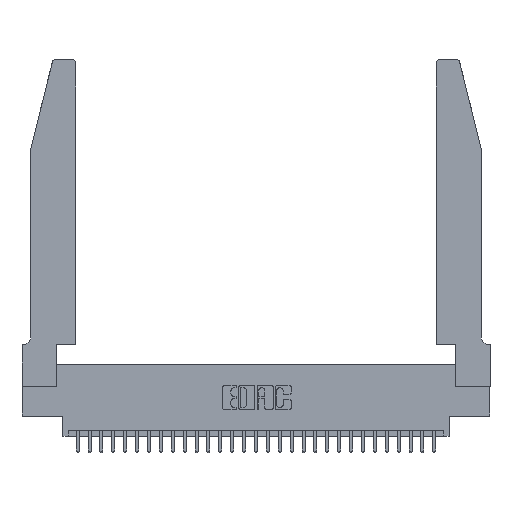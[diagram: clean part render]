
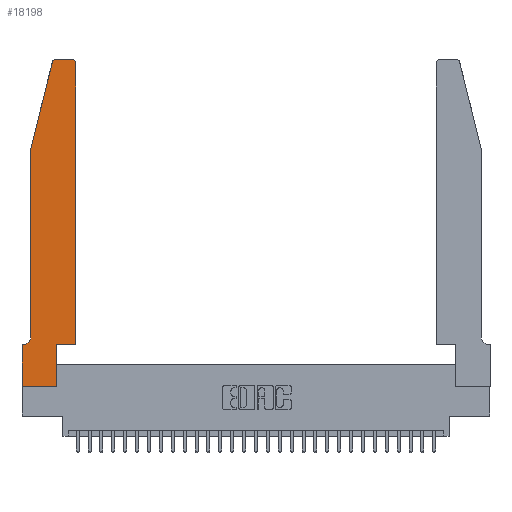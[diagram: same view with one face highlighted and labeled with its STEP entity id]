
A CAD part, top view. The second image highlights one B-rep face of the part: STEP entity #18198.
In plain terms, the highlighted planar face has unit normal (0, 0, 1).
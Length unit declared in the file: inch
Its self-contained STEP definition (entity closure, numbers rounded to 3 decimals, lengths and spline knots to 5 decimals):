
#87 = ORIENTED_EDGE ( 'NONE', *, *, #26610, .T. ) ;
#181 = EDGE_CURVE ( 'NONE', #12539, #19813, #25305, .T. ) ;
#554 = DIRECTION ( 'NONE',  ( -1., 0., 0. ) ) ;
#664 = VERTEX_POINT ( 'NONE', #16777 ) ;
#1028 = CARTESIAN_POINT ( 'NONE',  ( 0.284, 2.72, 0.37 ) ) ;
#1077 = VECTOR ( 'NONE', #25395, 39.37008 ) ;
#1329 = DIRECTION ( 'NONE',  ( 0., -1., 0. ) ) ;
#1343 = AXIS2_PLACEMENT_3D ( 'NONE', #1028, #15562, #18183 ) ;
#1642 = PLANE ( 'NONE',  #27642 ) ;
#1936 = VECTOR ( 'NONE', #29072, 39.37008 ) ;
#2067 = VECTOR ( 'NONE', #19084, 39.37008 ) ;
#2188 = EDGE_CURVE ( 'NONE', #20248, #12539, #9229, .T. ) ;
#2375 = CARTESIAN_POINT ( 'NONE',  ( 0.2605, 2.75, 0.37 ) ) ;
#2540 = EDGE_CURVE ( 'NONE', #14638, #664, #21098, .T. ) ;
#2846 = CARTESIAN_POINT ( 'NONE',  ( 0.0755, 0.42, 0.37 ) ) ;
#2885 = DIRECTION ( 'NONE',  ( 0., 0., -1. ) ) ;
#3197 = LINE ( 'NONE', #24258, #2067 ) ;
#3876 = ORIENTED_EDGE ( 'NONE', *, *, #10093, .T. ) ;
#4093 = CARTESIAN_POINT ( 'NONE',  ( 0.2865, 0., 0.37 ) ) ;
#4154 = CARTESIAN_POINT ( 'NONE',  ( 0., 0.35, 0.37 ) ) ;
#4355 = VERTEX_POINT ( 'NONE', #4093 ) ;
#4434 = ORIENTED_EDGE ( 'NONE', *, *, #7780, .T. ) ;
#4638 = EDGE_CURVE ( 'NONE', #12051, #20248, #3197, .T. ) ;
#5009 = VECTOR ( 'NONE', #9627, 39.37008 ) ;
#6505 = CARTESIAN_POINT ( 'NONE',  ( 0., 0., 0.37 ) ) ;
#6773 = ORIENTED_EDGE ( 'NONE', *, *, #2188, .T. ) ;
#7277 = LINE ( 'NONE', #15539, #18431 ) ;
#7606 = VERTEX_POINT ( 'NONE', #23013 ) ;
#7780 = EDGE_CURVE ( 'NONE', #11461, #8912, #7277, .T. ) ;
#8151 = FACE_OUTER_BOUND ( 'NONE', #8646, .T. ) ;
#8602 = VECTOR ( 'NONE', #15467, 39.37008 ) ;
#8646 = EDGE_LOOP ( 'NONE', ( #18531, #27250, #12025, #4434, #87, #20760, #17244, #13433, #3876, #18846, #6773, #12962 ) ) ;
#8819 = CARTESIAN_POINT ( 'NONE',  ( 0.2865, 0.35, 0.37 ) ) ;
#8910 = LINE ( 'NONE', #6505, #1077 ) ;
#8912 = VERTEX_POINT ( 'NONE', #2846 ) ;
#9094 = LINE ( 'NONE', #2375, #5009 ) ;
#9229 = LINE ( 'NONE', #27518, #27403 ) ;
#9627 = DIRECTION ( 'NONE',  ( -1., 0., 0. ) ) ;
#9867 = CARTESIAN_POINT ( 'NONE',  ( 0.4505, 0.35, 0.37 ) ) ;
#10080 = LINE ( 'NONE', #29781, #8602 ) ;
#10093 = EDGE_CURVE ( 'NONE', #4355, #12051, #19071, .T. ) ;
#10514 = CARTESIAN_POINT ( 'NONE',  ( 0.0755, 2., 0.37 ) ) ;
#11186 = EDGE_CURVE ( 'NONE', #20936, #7606, #16382, .T. ) ;
#11461 = VERTEX_POINT ( 'NONE', #28165 ) ;
#12025 = ORIENTED_EDGE ( 'NONE', *, *, #25630, .T. ) ;
#12051 = VERTEX_POINT ( 'NONE', #16110 ) ;
#12072 = CARTESIAN_POINT ( 'NONE',  ( 0.284, 2.75, 0.37 ) ) ;
#12432 = CARTESIAN_POINT ( 'NONE',  ( 0.4505, 2.72, 0.37 ) ) ;
#12539 = VERTEX_POINT ( 'NONE', #12432 ) ;
#12833 = CARTESIAN_POINT ( 'NONE',  ( 0.0055, 0.35, 0.37 ) ) ;
#12962 = ORIENTED_EDGE ( 'NONE', *, *, #181, .T. ) ;
#13433 = ORIENTED_EDGE ( 'NONE', *, *, #26875, .T. ) ;
#13612 = DIRECTION ( 'NONE',  ( 1., 0., 0. ) ) ;
#13752 = DIRECTION ( 'NONE',  ( 0., 1., 0. ) ) ;
#14054 = DIRECTION ( 'NONE',  ( 0., -1., 0. ) ) ;
#14638 = VERTEX_POINT ( 'NONE', #12072 ) ;
#14812 = CARTESIAN_POINT ( 'NONE',  ( 0.0055, 0.42, 0.37 ) ) ;
#15467 = DIRECTION ( 'NONE',  ( -1., 0., 0. ) ) ;
#15539 = CARTESIAN_POINT ( 'NONE',  ( 0.0755, 2., 0.37 ) ) ;
#15562 = DIRECTION ( 'NONE',  ( 0., 0., 1. ) ) ;
#16110 = CARTESIAN_POINT ( 'NONE',  ( 0.2865, 0.35, 0.37 ) ) ;
#16177 = CARTESIAN_POINT ( 'NONE',  ( 0., 0.35, 0.37 ) ) ;
#16191 = DIRECTION ( 'NONE',  ( 0., 0., 1. ) ) ;
#16382 = LINE ( 'NONE', #25658, #18257 ) ;
#16777 = CARTESIAN_POINT ( 'NONE',  ( 0.25487, 2.72718, 0.37 ) ) ;
#17244 = ORIENTED_EDGE ( 'NONE', *, *, #11186, .T. ) ;
#17382 = CARTESIAN_POINT ( 'NONE',  ( 0.4205, 2.75, 0.37 ) ) ;
#18183 = DIRECTION ( 'NONE',  ( 1., 0., 0. ) ) ;
#18198 = ADVANCED_FACE ( 'NONE', ( #8151 ), #1642, .T. ) ;
#18257 = VECTOR ( 'NONE', #14054, 39.37008 ) ;
#18431 = VECTOR ( 'NONE', #1329, 39.37008 ) ;
#18531 = ORIENTED_EDGE ( 'NONE', *, *, #30310, .T. ) ;
#18602 = DIRECTION ( 'NONE',  ( 1., 0., 0. ) ) ;
#18846 = ORIENTED_EDGE ( 'NONE', *, *, #4638, .T. ) ;
#19062 = LINE ( 'NONE', #10514, #1936 ) ;
#19071 = LINE ( 'NONE', #8819, #26088 ) ;
#19084 = DIRECTION ( 'NONE',  ( 1., 0., 0. ) ) ;
#19813 = VERTEX_POINT ( 'NONE', #17382 ) ;
#20248 = VERTEX_POINT ( 'NONE', #9867 ) ;
#20760 = ORIENTED_EDGE ( 'NONE', *, *, #25835, .T. ) ;
#20936 = VERTEX_POINT ( 'NONE', #4154 ) ;
#21098 = CIRCLE ( 'NONE', #1343, 0.03 ) ;
#23013 = CARTESIAN_POINT ( 'NONE',  ( 0., 0., 0.37 ) ) ;
#23572 = CARTESIAN_POINT ( 'NONE',  ( 0.4205, 2.72, 0.37 ) ) ;
#23743 = AXIS2_PLACEMENT_3D ( 'NONE', #23572, #16191, #18602 ) ;
#24258 = CARTESIAN_POINT ( 'NONE',  ( 0.4505, 0.35, 0.37 ) ) ;
#25096 = AXIS2_PLACEMENT_3D ( 'NONE', #14812, #2885, #554 ) ;
#25305 = CIRCLE ( 'NONE', #23743, 0.03 ) ;
#25395 = DIRECTION ( 'NONE',  ( 1., 0., 0. ) ) ;
#25630 = EDGE_CURVE ( 'NONE', #664, #11461, #19062, .T. ) ;
#25658 = CARTESIAN_POINT ( 'NONE',  ( 0., 0., 0.37 ) ) ;
#25835 = EDGE_CURVE ( 'NONE', #26753, #20936, #10080, .T. ) ;
#26088 = VECTOR ( 'NONE', #30190, 39.37008 ) ;
#26610 = EDGE_CURVE ( 'NONE', #8912, #26753, #28952, .T. ) ;
#26753 = VERTEX_POINT ( 'NONE', #12833 ) ;
#26875 = EDGE_CURVE ( 'NONE', #7606, #4355, #8910, .T. ) ;
#27250 = ORIENTED_EDGE ( 'NONE', *, *, #2540, .T. ) ;
#27403 = VECTOR ( 'NONE', #13752, 39.37008 ) ;
#27518 = CARTESIAN_POINT ( 'NONE',  ( 0.4505, 0.35, 0.37 ) ) ;
#27642 = AXIS2_PLACEMENT_3D ( 'NONE', #16177, #27907, #13612 ) ;
#27907 = DIRECTION ( 'NONE',  ( 0., 0., 1. ) ) ;
#28165 = CARTESIAN_POINT ( 'NONE',  ( 0.0755, 2., 0.37 ) ) ;
#28952 = CIRCLE ( 'NONE', #25096, 0.07 ) ;
#29072 = DIRECTION ( 'NONE',  ( -0.239, -0.971, 0. ) ) ;
#29781 = CARTESIAN_POINT ( 'NONE',  ( 0.0755, 0.35, 0.37 ) ) ;
#30190 = DIRECTION ( 'NONE',  ( 0., 1., 0. ) ) ;
#30310 = EDGE_CURVE ( 'NONE', #19813, #14638, #9094, .T. ) ;
